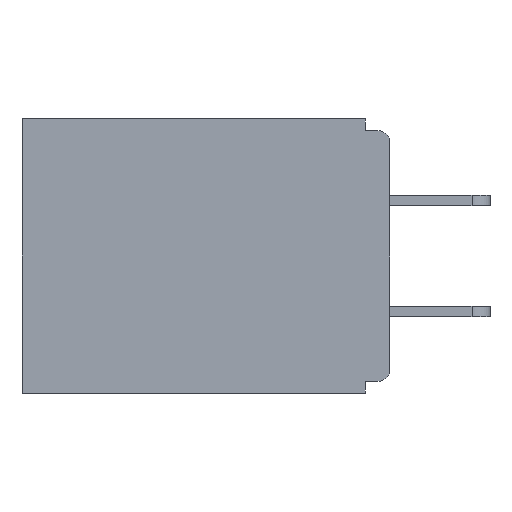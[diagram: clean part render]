
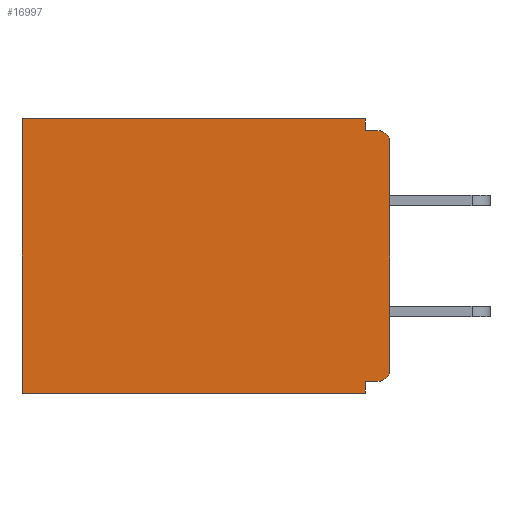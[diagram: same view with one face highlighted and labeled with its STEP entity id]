
A CAD part, left-side view. The second image highlights one B-rep face of the part: STEP entity #16997.
In plain terms, the highlighted planar face has unit normal (-1, 0, 0).
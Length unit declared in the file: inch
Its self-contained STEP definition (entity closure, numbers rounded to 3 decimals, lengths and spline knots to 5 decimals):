
#153 = LINE ( 'NONE', #13285, #29579 ) ;
#533 = CARTESIAN_POINT ( 'NONE',  ( 0.298, 0., 0. ) ) ;
#1556 = VERTEX_POINT ( 'NONE', #11867 ) ;
#1598 = VERTEX_POINT ( 'NONE', #16600 ) ;
#2313 = CARTESIAN_POINT ( 'NONE',  ( 0.298, 0., -0.313 ) ) ;
#2365 = VECTOR ( 'NONE', #18379, 39.37008 ) ;
#2961 = VERTEX_POINT ( 'NONE', #2313 ) ;
#3726 = VERTEX_POINT ( 'NONE', #5664 ) ;
#4999 = DIRECTION ( 'NONE',  ( 0., 0., -1. ) ) ;
#5225 = PLANE ( 'NONE',  #14566 ) ;
#5253 = DIRECTION ( 'NONE',  ( 0., 1., 0. ) ) ;
#5416 = CARTESIAN_POINT ( 'NONE',  ( 0.298, 0.46, -0.343 ) ) ;
#5442 = CIRCLE ( 'NONE', #25702, 0.015 ) ;
#5597 = EDGE_CURVE ( 'NONE', #1556, #13580, #6520, .T. ) ;
#5664 = CARTESIAN_POINT ( 'NONE',  ( 0.298, 0.031, -0.343 ) ) ;
#5971 = ORIENTED_EDGE ( 'NONE', *, *, #8451, .F. ) ;
#6103 = ORIENTED_EDGE ( 'NONE', *, *, #23110, .T. ) ;
#6520 = LINE ( 'NONE', #8300, #11869 ) ;
#6692 = LINE ( 'NONE', #7363, #22827 ) ;
#7363 = CARTESIAN_POINT ( 'NONE',  ( 0.298, 0.031, -0.343 ) ) ;
#8200 = VECTOR ( 'NONE', #20696, 39.37008 ) ;
#8300 = CARTESIAN_POINT ( 'NONE',  ( 0.298, 0., -0.015 ) ) ;
#8451 = EDGE_CURVE ( 'NONE', #26435, #1556, #6692, .T. ) ;
#9315 = CARTESIAN_POINT ( 'NONE',  ( 0.298, 0.015, -0.328 ) ) ;
#9646 = EDGE_CURVE ( 'NONE', #26435, #1598, #23162, .T. ) ;
#9705 = DIRECTION ( 'NONE',  ( 0., 0., -1. ) ) ;
#10221 = EDGE_CURVE ( 'NONE', #23874, #27640, #153, .T. ) ;
#10845 = FACE_OUTER_BOUND ( 'NONE', #17999, .T. ) ;
#11373 = ORIENTED_EDGE ( 'NONE', *, *, #12670, .T. ) ;
#11867 = CARTESIAN_POINT ( 'NONE',  ( 0.298, 0.031, -0.015 ) ) ;
#11869 = VECTOR ( 'NONE', #12926, 39.37008 ) ;
#12416 = DIRECTION ( 'NONE',  ( -1., 0., 0. ) ) ;
#12545 = CARTESIAN_POINT ( 'NONE',  ( 0.298, 0.46, 0. ) ) ;
#12569 = CARTESIAN_POINT ( 'NONE',  ( 0.298, 0.031, -0.328 ) ) ;
#12646 = VERTEX_POINT ( 'NONE', #14723 ) ;
#12670 = EDGE_CURVE ( 'NONE', #23874, #2961, #5442, .T. ) ;
#12926 = DIRECTION ( 'NONE',  ( 0., -1., 0. ) ) ;
#13285 = CARTESIAN_POINT ( 'NONE',  ( 0.298, 0., -0.328 ) ) ;
#13367 = EDGE_CURVE ( 'NONE', #3726, #14664, #14656, .T. ) ;
#13580 = VERTEX_POINT ( 'NONE', #15599 ) ;
#14013 = EDGE_CURVE ( 'NONE', #1598, #14664, #21493, .T. ) ;
#14312 = DIRECTION ( 'NONE',  ( 1., 0., 0. ) ) ;
#14566 = AXIS2_PLACEMENT_3D ( 'NONE', #533, #14312, #9705 ) ;
#14656 = LINE ( 'NONE', #14825, #27603 ) ;
#14664 = VERTEX_POINT ( 'NONE', #5416 ) ;
#14723 = CARTESIAN_POINT ( 'NONE',  ( 0.298, 0., -0.03 ) ) ;
#14822 = ORIENTED_EDGE ( 'NONE', *, *, #5597, .F. ) ;
#14825 = CARTESIAN_POINT ( 'NONE',  ( 0.298, 0., -0.343 ) ) ;
#15388 = CARTESIAN_POINT ( 'NONE',  ( 0.298, 0.031, 0. ) ) ;
#15599 = CARTESIAN_POINT ( 'NONE',  ( 0.298, 0.015, -0.015 ) ) ;
#15661 = CARTESIAN_POINT ( 'NONE',  ( 0.298, 0., 0. ) ) ;
#16600 = CARTESIAN_POINT ( 'NONE',  ( 0.298, 0.46, 0. ) ) ;
#16943 = DIRECTION ( 'NONE',  ( 0., 0., -1. ) ) ;
#16997 = ADVANCED_FACE ( 'NONE', ( #10845 ), #5225, .F. ) ;
#17999 = EDGE_LOOP ( 'NONE', ( #6103, #14822, #5971, #22602, #22192, #22657, #29120, #20828, #11373, #20195 ) ) ;
#18379 = DIRECTION ( 'NONE',  ( 0., 1., 0. ) ) ;
#18719 = AXIS2_PLACEMENT_3D ( 'NONE', #23251, #25579, #4999 ) ;
#19154 = DIRECTION ( 'NONE',  ( 0., 0., -1. ) ) ;
#19683 = EDGE_CURVE ( 'NONE', #27640, #3726, #22413, .T. ) ;
#20195 = ORIENTED_EDGE ( 'NONE', *, *, #24546, .F. ) ;
#20411 = CIRCLE ( 'NONE', #18719, 0.015 ) ;
#20696 = DIRECTION ( 'NONE',  ( 0., 0., -1. ) ) ;
#20828 = ORIENTED_EDGE ( 'NONE', *, *, #10221, .F. ) ;
#21356 = VECTOR ( 'NONE', #16943, 39.37008 ) ;
#21493 = LINE ( 'NONE', #12545, #27578 ) ;
#22192 = ORIENTED_EDGE ( 'NONE', *, *, #14013, .T. ) ;
#22413 = LINE ( 'NONE', #24015, #21356 ) ;
#22602 = ORIENTED_EDGE ( 'NONE', *, *, #9646, .T. ) ;
#22657 = ORIENTED_EDGE ( 'NONE', *, *, #13367, .F. ) ;
#22787 = CARTESIAN_POINT ( 'NONE',  ( 0.298, 0., 0. ) ) ;
#22827 = VECTOR ( 'NONE', #19154, 39.37008 ) ;
#23110 = EDGE_CURVE ( 'NONE', #12646, #13580, #20411, .T. ) ;
#23162 = LINE ( 'NONE', #15661, #2365 ) ;
#23251 = CARTESIAN_POINT ( 'NONE',  ( 0.298, 0.015, -0.03 ) ) ;
#23874 = VERTEX_POINT ( 'NONE', #9315 ) ;
#24015 = CARTESIAN_POINT ( 'NONE',  ( 0.298, 0.031, -0.343 ) ) ;
#24546 = EDGE_CURVE ( 'NONE', #12646, #2961, #28634, .T. ) ;
#24782 = DIRECTION ( 'NONE',  ( 0., 1., 0. ) ) ;
#25579 = DIRECTION ( 'NONE',  ( -1., 0., 0. ) ) ;
#25702 = AXIS2_PLACEMENT_3D ( 'NONE', #28379, #12416, #28491 ) ;
#26231 = DIRECTION ( 'NONE',  ( 0., 0., -1. ) ) ;
#26435 = VERTEX_POINT ( 'NONE', #15388 ) ;
#27578 = VECTOR ( 'NONE', #26231, 39.37008 ) ;
#27603 = VECTOR ( 'NONE', #5253, 39.37008 ) ;
#27640 = VERTEX_POINT ( 'NONE', #12569 ) ;
#28379 = CARTESIAN_POINT ( 'NONE',  ( 0.298, 0.015, -0.313 ) ) ;
#28491 = DIRECTION ( 'NONE',  ( 0., 0., -1. ) ) ;
#28634 = LINE ( 'NONE', #22787, #8200 ) ;
#29120 = ORIENTED_EDGE ( 'NONE', *, *, #19683, .F. ) ;
#29579 = VECTOR ( 'NONE', #24782, 39.37008 ) ;
